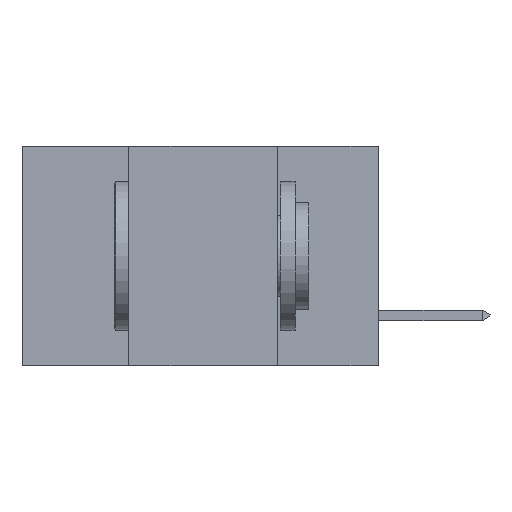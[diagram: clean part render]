
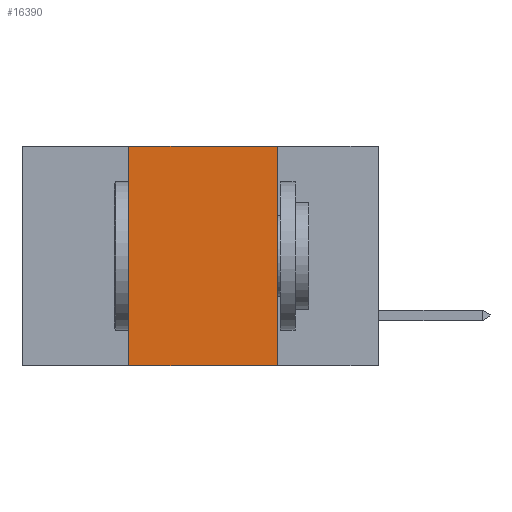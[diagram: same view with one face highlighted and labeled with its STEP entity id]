
A CAD part, left-side view. The second image highlights one B-rep face of the part: STEP entity #16390.
In plain terms, the highlighted planar face has unit normal (-1, 0, 0).
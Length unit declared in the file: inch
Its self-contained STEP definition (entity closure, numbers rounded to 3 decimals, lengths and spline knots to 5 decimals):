
#237 = DIRECTION ( 'NONE',  ( 0., 0., -1. ) ) ;
#657 = LINE ( 'NONE', #10534, #22829 ) ;
#985 = LINE ( 'NONE', #4517, #20524 ) ;
#1399 = CARTESIAN_POINT ( 'NONE',  ( 0., 0.6, 0. ) ) ;
#3339 = FACE_OUTER_BOUND ( 'NONE', #20050, .T. ) ;
#4017 = LINE ( 'NONE', #18041, #15695 ) ;
#4517 = CARTESIAN_POINT ( 'NONE',  ( 0., 0.6, 0. ) ) ;
#4921 = ORIENTED_EDGE ( 'NONE', *, *, #20876, .F. ) ;
#4956 = EDGE_CURVE ( 'NONE', #18259, #7464, #4017, .T. ) ;
#6475 = EDGE_CURVE ( 'NONE', #11906, #7464, #17171, .T. ) ;
#7464 = VERTEX_POINT ( 'NONE', #17399 ) ;
#10534 = CARTESIAN_POINT ( 'NONE',  ( 0., 0.42, -0.37 ) ) ;
#11187 = VECTOR ( 'NONE', #19378, 39.37008 ) ;
#11417 = PLANE ( 'NONE',  #12953 ) ;
#11906 = VERTEX_POINT ( 'NONE', #24685 ) ;
#12351 = DIRECTION ( 'NONE',  ( 0., 0., 1. ) ) ;
#12953 = AXIS2_PLACEMENT_3D ( 'NONE', #1399, #15031, #18932 ) ;
#13272 = CARTESIAN_POINT ( 'NONE',  ( 0., 0.6, -0.37 ) ) ;
#14285 = ORIENTED_EDGE ( 'NONE', *, *, #6475, .T. ) ;
#14641 = DIRECTION ( 'NONE',  ( 0., -1., 0. ) ) ;
#15031 = DIRECTION ( 'NONE',  ( 1., 0., 0. ) ) ;
#15564 = CARTESIAN_POINT ( 'NONE',  ( 0., 0.17, 0. ) ) ;
#15695 = VECTOR ( 'NONE', #237, 39.37008 ) ;
#15704 = ORIENTED_EDGE ( 'NONE', *, *, #21580, .F. ) ;
#16390 = ADVANCED_FACE ( 'NONE', ( #3339 ), #11417, .F. ) ;
#17171 = LINE ( 'NONE', #13272, #11187 ) ;
#17399 = CARTESIAN_POINT ( 'NONE',  ( 0., 0.17, -0.37 ) ) ;
#18041 = CARTESIAN_POINT ( 'NONE',  ( 0., 0.17, -0.37 ) ) ;
#18096 = CARTESIAN_POINT ( 'NONE',  ( 0., 0.42, 0. ) ) ;
#18259 = VERTEX_POINT ( 'NONE', #15564 ) ;
#18932 = DIRECTION ( 'NONE',  ( 0., 0., -1. ) ) ;
#19378 = DIRECTION ( 'NONE',  ( 0., -1., 0. ) ) ;
#20050 = EDGE_LOOP ( 'NONE', ( #23099, #4921, #15704, #14285 ) ) ;
#20524 = VECTOR ( 'NONE', #14641, 39.37008 ) ;
#20876 = EDGE_CURVE ( 'NONE', #23416, #18259, #985, .T. ) ;
#21580 = EDGE_CURVE ( 'NONE', #11906, #23416, #657, .T. ) ;
#22829 = VECTOR ( 'NONE', #12351, 39.37008 ) ;
#23099 = ORIENTED_EDGE ( 'NONE', *, *, #4956, .F. ) ;
#23416 = VERTEX_POINT ( 'NONE', #18096 ) ;
#24685 = CARTESIAN_POINT ( 'NONE',  ( 0., 0.42, -0.37 ) ) ;
